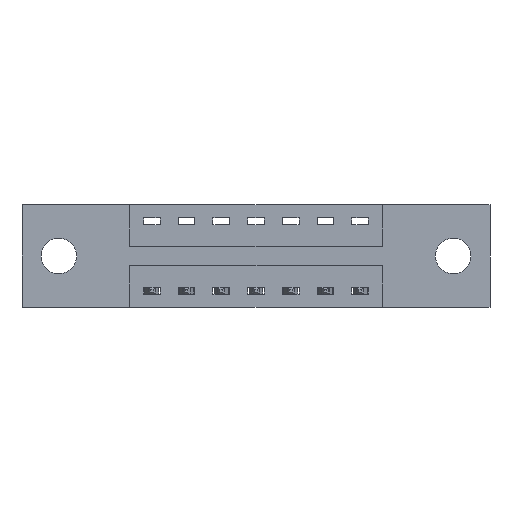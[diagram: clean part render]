
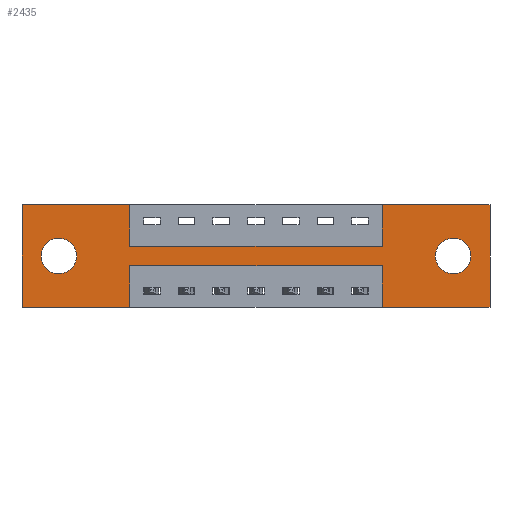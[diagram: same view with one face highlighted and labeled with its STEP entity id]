
A CAD part, front view. The second image highlights one B-rep face of the part: STEP entity #2435.
In plain terms, the highlighted planar face has unit normal (0, -1, 0).
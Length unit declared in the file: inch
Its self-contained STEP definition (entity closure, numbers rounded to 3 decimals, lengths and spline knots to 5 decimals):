
#105 = VERTEX_POINT ( 'NONE', #7953 ) ;
#185 = VERTEX_POINT ( 'NONE', #7002 ) ;
#234 = VERTEX_POINT ( 'NONE', #823 ) ;
#273 = LINE ( 'NONE', #7460, #7451 ) ;
#304 = EDGE_CURVE ( 'NONE', #1520, #8413, #4708, .T. ) ;
#414 = DIRECTION ( 'NONE',  ( 0., 1., 0. ) ) ;
#416 = VERTEX_POINT ( 'NONE', #5239 ) ;
#421 = ORIENTED_EDGE ( 'NONE', *, *, #6766, .F. ) ;
#426 = ORIENTED_EDGE ( 'NONE', *, *, #6760, .F. ) ;
#539 = CARTESIAN_POINT ( 'NONE',  ( 0.3875, 0., 0. ) ) ;
#584 = ORIENTED_EDGE ( 'NONE', *, *, #6587, .F. ) ;
#823 = CARTESIAN_POINT ( 'NONE',  ( 0.3875, 0., -0.22 ) ) ;
#853 = ORIENTED_EDGE ( 'NONE', *, *, #3539, .F. ) ;
#912 = CARTESIAN_POINT ( 'NONE',  ( 0., 0., -0.37 ) ) ;
#975 = FACE_BOUND ( 'NONE', #1273, .T. ) ;
#1061 = DIRECTION ( 'NONE',  ( -1., 0., 0. ) ) ;
#1273 = EDGE_LOOP ( 'NONE', ( #4239, #5025 ) ) ;
#1279 = CARTESIAN_POINT ( 'NONE',  ( 1.2975, 0., -0.37 ) ) ;
#1367 = LINE ( 'NONE', #7884, #5208 ) ;
#1395 = ORIENTED_EDGE ( 'NONE', *, *, #7781, .F. ) ;
#1460 = AXIS2_PLACEMENT_3D ( 'NONE', #2537, #414, #3873 ) ;
#1487 = CARTESIAN_POINT ( 'NONE',  ( 1.2975, 0., -0.37 ) ) ;
#1520 = VERTEX_POINT ( 'NONE', #2241 ) ;
#1528 = AXIS2_PLACEMENT_3D ( 'NONE', #6871, #2570, #7572 ) ;
#1621 = LINE ( 'NONE', #5858, #5234 ) ;
#1684 = VECTOR ( 'NONE', #8933, 39.37008 ) ;
#1757 = LINE ( 'NONE', #3297, #5584 ) ;
#1805 = VERTEX_POINT ( 'NONE', #7352 ) ;
#1966 = EDGE_CURVE ( 'NONE', #105, #5264, #8258, .T. ) ;
#2123 = AXIS2_PLACEMENT_3D ( 'NONE', #7084, #6576, #4050 ) ;
#2127 = DIRECTION ( 'NONE',  ( -1., 0., 0. ) ) ;
#2183 = VERTEX_POINT ( 'NONE', #8673 ) ;
#2241 = CARTESIAN_POINT ( 'NONE',  ( 0.1325, 0., -0.121 ) ) ;
#2322 = VERTEX_POINT ( 'NONE', #4612 ) ;
#2399 = ORIENTED_EDGE ( 'NONE', *, *, #4583, .F. ) ;
#2435 = ADVANCED_FACE ( 'NONE', ( #6904, #975, #4793 ), #6519, .T. ) ;
#2438 = VECTOR ( 'NONE', #4385, 39.37008 ) ;
#2484 = CARTESIAN_POINT ( 'NONE',  ( 0., 0., -0.37 ) ) ;
#2537 = CARTESIAN_POINT ( 'NONE',  ( 1.5525, 0., -0.185 ) ) ;
#2570 = DIRECTION ( 'NONE',  ( 0., 1., 0. ) ) ;
#2738 = VECTOR ( 'NONE', #2914, 39.37008 ) ;
#2818 = CARTESIAN_POINT ( 'NONE',  ( 1.2975, 0., -0.15 ) ) ;
#2914 = DIRECTION ( 'NONE',  ( 0., 0., 1. ) ) ;
#2934 = ORIENTED_EDGE ( 'NONE', *, *, #3236, .T. ) ;
#3009 = DIRECTION ( 'NONE',  ( 0., 0., 1. ) ) ;
#3144 = CARTESIAN_POINT ( 'NONE',  ( 0., 0., -0.37 ) ) ;
#3178 = DIRECTION ( 'NONE',  ( 1., 0., 0. ) ) ;
#3236 = EDGE_CURVE ( 'NONE', #3806, #2322, #5874, .T. ) ;
#3250 = VERTEX_POINT ( 'NONE', #7751 ) ;
#3294 = EDGE_CURVE ( 'NONE', #5902, #105, #1621, .T. ) ;
#3297 = CARTESIAN_POINT ( 'NONE',  ( 0., 0., 0. ) ) ;
#3425 = VECTOR ( 'NONE', #1061, 39.37008 ) ;
#3510 = EDGE_CURVE ( 'NONE', #2322, #3806, #3653, .T. ) ;
#3539 = EDGE_CURVE ( 'NONE', #4117, #416, #8327, .T. ) ;
#3581 = DIRECTION ( 'NONE',  ( 0., 0., -1. ) ) ;
#3653 = CIRCLE ( 'NONE', #1460, 0.064 ) ;
#3680 = DIRECTION ( 'NONE',  ( 1., 0., 0. ) ) ;
#3788 = LINE ( 'NONE', #9043, #9070 ) ;
#3806 = VERTEX_POINT ( 'NONE', #5641 ) ;
#3873 = DIRECTION ( 'NONE',  ( 0., 0., -1. ) ) ;
#3979 = ORIENTED_EDGE ( 'NONE', *, *, #3510, .T. ) ;
#4050 = DIRECTION ( 'NONE',  ( 0., 0., -1. ) ) ;
#4109 = AXIS2_PLACEMENT_3D ( 'NONE', #5533, #8817, #7110 ) ;
#4117 = VERTEX_POINT ( 'NONE', #3144 ) ;
#4239 = ORIENTED_EDGE ( 'NONE', *, *, #304, .T. ) ;
#4260 = CARTESIAN_POINT ( 'NONE',  ( 0., 0., 0. ) ) ;
#4337 = LINE ( 'NONE', #5777, #2438 ) ;
#4385 = DIRECTION ( 'NONE',  ( -1., 0., 0. ) ) ;
#4583 = EDGE_CURVE ( 'NONE', #185, #8180, #1367, .T. ) ;
#4612 = CARTESIAN_POINT ( 'NONE',  ( 1.5525, 0., -0.249 ) ) ;
#4708 = CIRCLE ( 'NONE', #7536, 0.064 ) ;
#4761 = LINE ( 'NONE', #7527, #8216 ) ;
#4793 = FACE_OUTER_BOUND ( 'NONE', #8513, .T. ) ;
#5025 = ORIENTED_EDGE ( 'NONE', *, *, #5575, .T. ) ;
#5208 = VECTOR ( 'NONE', #3680, 39.37008 ) ;
#5234 = VECTOR ( 'NONE', #3581, 39.37008 ) ;
#5239 = CARTESIAN_POINT ( 'NONE',  ( 0., 0., 0. ) ) ;
#5264 = VERTEX_POINT ( 'NONE', #1487 ) ;
#5343 = LINE ( 'NONE', #2484, #3425 ) ;
#5401 = DIRECTION ( 'NONE',  ( 0., 0., -1. ) ) ;
#5434 = ORIENTED_EDGE ( 'NONE', *, *, #8753, .F. ) ;
#5470 = VECTOR ( 'NONE', #9013, 39.37008 ) ;
#5512 = LINE ( 'NONE', #1279, #1684 ) ;
#5533 = CARTESIAN_POINT ( 'NONE',  ( 0., 0., -0.37 ) ) ;
#5575 = EDGE_CURVE ( 'NONE', #8413, #1520, #6392, .T. ) ;
#5584 = VECTOR ( 'NONE', #8188, 39.37008 ) ;
#5641 = CARTESIAN_POINT ( 'NONE',  ( 1.5525, 0., -0.121 ) ) ;
#5658 = DIRECTION ( 'NONE',  ( 0., 0., 1. ) ) ;
#5710 = EDGE_CURVE ( 'NONE', #5264, #3250, #5512, .T. ) ;
#5777 = CARTESIAN_POINT ( 'NONE',  ( 0.3875, 0., -0.22 ) ) ;
#5858 = CARTESIAN_POINT ( 'NONE',  ( 1.685, 0., 0. ) ) ;
#5874 = CIRCLE ( 'NONE', #2123, 0.064 ) ;
#5893 = LINE ( 'NONE', #8379, #5470 ) ;
#5902 = VERTEX_POINT ( 'NONE', #7180 ) ;
#6017 = CARTESIAN_POINT ( 'NONE',  ( 0.1325, 0., -0.185 ) ) ;
#6089 = DIRECTION ( 'NONE',  ( 0., 1., 0. ) ) ;
#6153 = ORIENTED_EDGE ( 'NONE', *, *, #6877, .F. ) ;
#6216 = VERTEX_POINT ( 'NONE', #539 ) ;
#6392 = CIRCLE ( 'NONE', #1528, 0.064 ) ;
#6470 = VECTOR ( 'NONE', #2127, 39.37008 ) ;
#6519 = PLANE ( 'NONE',  #4109 ) ;
#6576 = DIRECTION ( 'NONE',  ( 0., 1., 0. ) ) ;
#6577 = ORIENTED_EDGE ( 'NONE', *, *, #5710, .F. ) ;
#6587 = EDGE_CURVE ( 'NONE', #416, #6216, #1757, .T. ) ;
#6760 = EDGE_CURVE ( 'NONE', #6216, #185, #5893, .T. ) ;
#6766 = EDGE_CURVE ( 'NONE', #8180, #2183, #3788, .T. ) ;
#6871 = CARTESIAN_POINT ( 'NONE',  ( 0.1325, 0., -0.185 ) ) ;
#6877 = EDGE_CURVE ( 'NONE', #3250, #234, #4337, .T. ) ;
#6895 = ORIENTED_EDGE ( 'NONE', *, *, #1966, .F. ) ;
#6904 = FACE_BOUND ( 'NONE', #7792, .T. ) ;
#7002 = CARTESIAN_POINT ( 'NONE',  ( 0.3875, 0., -0.15 ) ) ;
#7084 = CARTESIAN_POINT ( 'NONE',  ( 1.5525, 0., -0.185 ) ) ;
#7110 = DIRECTION ( 'NONE',  ( 0., 0., -1. ) ) ;
#7180 = CARTESIAN_POINT ( 'NONE',  ( 1.685, 0., 0. ) ) ;
#7287 = ORIENTED_EDGE ( 'NONE', *, *, #3294, .F. ) ;
#7352 = CARTESIAN_POINT ( 'NONE',  ( 0.3875, 0., -0.37 ) ) ;
#7451 = VECTOR ( 'NONE', #3178, 39.37008 ) ;
#7460 = CARTESIAN_POINT ( 'NONE',  ( 0., 0., 0. ) ) ;
#7527 = CARTESIAN_POINT ( 'NONE',  ( 0.3875, 0., -0.37 ) ) ;
#7536 = AXIS2_PLACEMENT_3D ( 'NONE', #6017, #6089, #3009 ) ;
#7572 = DIRECTION ( 'NONE',  ( 0., 0., 1. ) ) ;
#7654 = ORIENTED_EDGE ( 'NONE', *, *, #7736, .F. ) ;
#7736 = EDGE_CURVE ( 'NONE', #2183, #5902, #273, .T. ) ;
#7751 = CARTESIAN_POINT ( 'NONE',  ( 1.2975, 0., -0.22 ) ) ;
#7781 = EDGE_CURVE ( 'NONE', #1805, #4117, #5343, .T. ) ;
#7792 = EDGE_LOOP ( 'NONE', ( #2934, #3979 ) ) ;
#7884 = CARTESIAN_POINT ( 'NONE',  ( 0.3875, 0., -0.15 ) ) ;
#7953 = CARTESIAN_POINT ( 'NONE',  ( 1.685, 0., -0.37 ) ) ;
#8180 = VERTEX_POINT ( 'NONE', #2818 ) ;
#8188 = DIRECTION ( 'NONE',  ( 1., 0., 0. ) ) ;
#8216 = VECTOR ( 'NONE', #5401, 39.37008 ) ;
#8258 = LINE ( 'NONE', #912, #6470 ) ;
#8327 = LINE ( 'NONE', #4260, #2738 ) ;
#8379 = CARTESIAN_POINT ( 'NONE',  ( 0.3875, 0., 0. ) ) ;
#8413 = VERTEX_POINT ( 'NONE', #8561 ) ;
#8513 = EDGE_LOOP ( 'NONE', ( #5434, #6153, #6577, #6895, #7287, #7654, #421, #2399, #426, #584, #853, #1395 ) ) ;
#8561 = CARTESIAN_POINT ( 'NONE',  ( 0.1325, 0., -0.249 ) ) ;
#8673 = CARTESIAN_POINT ( 'NONE',  ( 1.2975, 0., 0. ) ) ;
#8753 = EDGE_CURVE ( 'NONE', #234, #1805, #4761, .T. ) ;
#8817 = DIRECTION ( 'NONE',  ( 0., -1., 0. ) ) ;
#8933 = DIRECTION ( 'NONE',  ( 0., 0., 1. ) ) ;
#9013 = DIRECTION ( 'NONE',  ( 0., 0., -1. ) ) ;
#9043 = CARTESIAN_POINT ( 'NONE',  ( 1.2975, 0., 0. ) ) ;
#9070 = VECTOR ( 'NONE', #5658, 39.37008 ) ;
